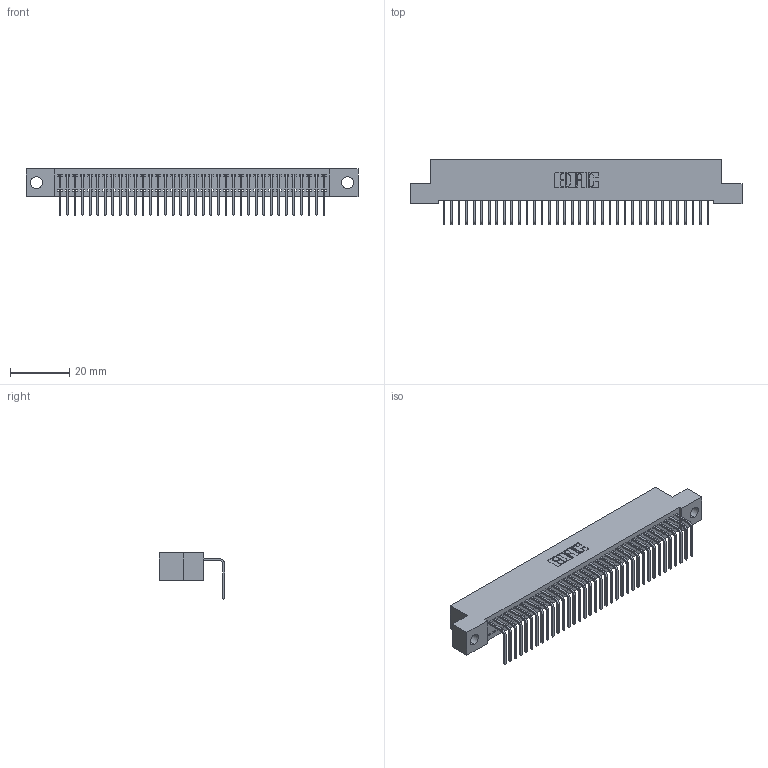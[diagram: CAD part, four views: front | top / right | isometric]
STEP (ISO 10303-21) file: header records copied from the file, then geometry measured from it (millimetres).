
FILE_DESCRIPTION (( 'STEP AP203' ), '1' );
FILE_NAME ('392-036-558-104.STEP', '2018-08-16T03:53:17', ( '' ), ( '' ), 'SwSTEP 2.0', 'SolidWorks 2016', '' );
FILE_SCHEMA (( 'CONFIG_CONTROL_DESIGN' ));
Length unit declared in the file: inch
Products named in the file (3): 342 Part_.156 TH; 345-292-001_558 Tail - 2; 392-036-558-104
Assembly tree (37 placements, depth 2):
  392-036-558-104
    342 Part_.156 TH
    345-292-001_558 Tail - 2  x36
Bounding box: 111.76 x 21.91 x 15.62 mm (x, y, z)
Volume: 9809.9 mm3; surface area: 14793.4 mm2
Topology: 37 solids, 37 shells, 2270 faces, 6851 edges, 4518 vertices
Faces by surface type: plane 1650, cylinder 620
Entity records: 22739 total; most frequent: CARTESIAN_POINT 3930, ORIENTED_EDGE 3902, DIRECTION 3327, EDGE_CURVE 1951, VECTOR 1823, LINE 1823, VERTEX_POINT 1298, AXIS2_PLACEMENT_3D 752
